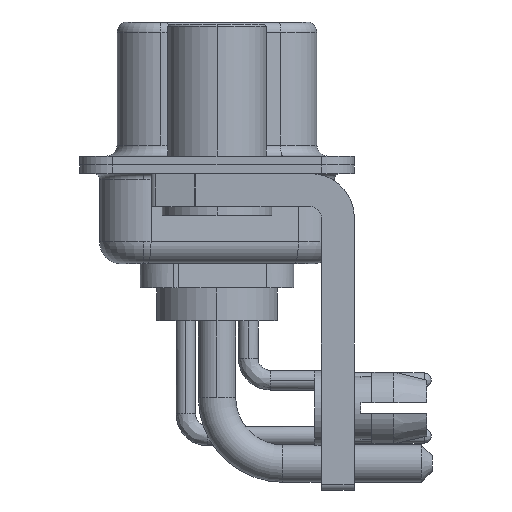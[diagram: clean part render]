
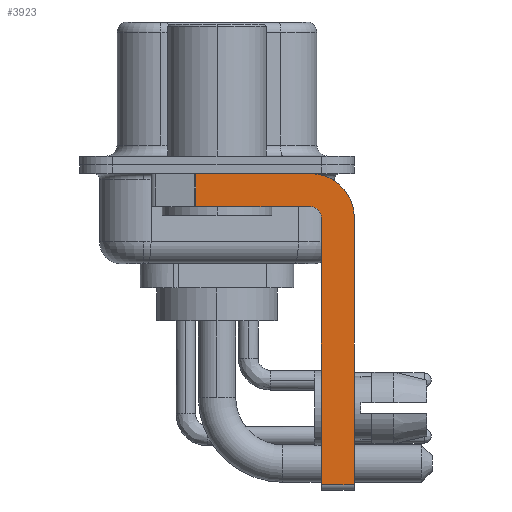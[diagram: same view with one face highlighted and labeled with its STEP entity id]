
A CAD part, left-side view. The second image highlights one B-rep face of the part: STEP entity #3923.
In plain terms, the highlighted planar face has unit normal (-1, 0, 0).
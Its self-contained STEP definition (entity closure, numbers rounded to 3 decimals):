
#31 = AXIS2_PLACEMENT_3D ( 'NONE', #22232, #9031, #4974 ) ;
#358 = VECTOR ( 'NONE', #23900, 1000. ) ;
#621 = EDGE_CURVE ( 'NONE', #6019, #10867, #24239, .T. ) ;
#1189 = LINE ( 'NONE', #20090, #23398 ) ;
#1366 = VERTEX_POINT ( 'NONE', #14848 ) ;
#1662 = DIRECTION ( 'NONE',  ( 0., 0., 1. ) ) ;
#2392 = AXIS2_PLACEMENT_3D ( 'NONE', #15628, #11678, #1662 ) ;
#2664 = LINE ( 'NONE', #11930, #7193 ) ;
#2903 = DIRECTION ( 'NONE',  ( 1., 0., 0. ) ) ;
#3574 = ORIENTED_EDGE ( 'NONE', *, *, #7593, .F. ) ;
#3923 = ADVANCED_FACE ( 'NONE', ( #22184 ), #6575, .F. ) ;
#4880 = CARTESIAN_POINT ( 'NONE',  ( -2.9, 3., -0.4 ) ) ;
#4974 = DIRECTION ( 'NONE',  ( 0., 0., -1. ) ) ;
#4986 = DIRECTION ( 'NONE',  ( 0., 1., 0. ) ) ;
#5110 = CARTESIAN_POINT ( 'NONE',  ( -2.9, -4.25, -1.9 ) ) ;
#5561 = DIRECTION ( 'NONE',  ( 0., 0., 1. ) ) ;
#6019 = VERTEX_POINT ( 'NONE', #6794 ) ;
#6575 = PLANE ( 'NONE',  #6641 ) ;
#6641 = AXIS2_PLACEMENT_3D ( 'NONE', #20277, #2903, #16482 ) ;
#6794 = CARTESIAN_POINT ( 'NONE',  ( -2.9, -4.75, -14.55 ) ) ;
#6993 = EDGE_CURVE ( 'NONE', #18891, #24413, #19817, .T. ) ;
#7193 = VECTOR ( 'NONE', #22077, 1000. ) ;
#7248 = EDGE_CURVE ( 'NONE', #1366, #14386, #2664, .T. ) ;
#7593 = EDGE_CURVE ( 'NONE', #6019, #18891, #18884, .T. ) ;
#8742 = ORIENTED_EDGE ( 'NONE', *, *, #6993, .F. ) ;
#9031 = DIRECTION ( 'NONE',  ( 1., 0., 0. ) ) ;
#9593 = CARTESIAN_POINT ( 'NONE',  ( -2.9, -4.75, -2.4 ) ) ;
#9919 = CARTESIAN_POINT ( 'NONE',  ( -2.9, -4.25, -0.4 ) ) ;
#10383 = ORIENTED_EDGE ( 'NONE', *, *, #7248, .T. ) ;
#10867 = VERTEX_POINT ( 'NONE', #16445 ) ;
#11344 = VECTOR ( 'NONE', #12627, 1000. ) ;
#11678 = DIRECTION ( 'NONE',  ( -1., 0., 0. ) ) ;
#11930 = CARTESIAN_POINT ( 'NONE',  ( -2.9, 0.978, -1.9 ) ) ;
#12595 = EDGE_CURVE ( 'NONE', #24413, #14386, #1189, .T. ) ;
#12627 = DIRECTION ( 'NONE',  ( 0., -1., 0. ) ) ;
#13892 = CARTESIAN_POINT ( 'NONE',  ( -2.9, -6.25, -2.4 ) ) ;
#13900 = ORIENTED_EDGE ( 'NONE', *, *, #19522, .F. ) ;
#14386 = VERTEX_POINT ( 'NONE', #22008 ) ;
#14742 = CARTESIAN_POINT ( 'NONE',  ( -2.9, -4.25, -14.55 ) ) ;
#14848 = CARTESIAN_POINT ( 'NONE',  ( -2.9, 0.978, -0.4 ) ) ;
#14945 = VERTEX_POINT ( 'NONE', #9919 ) ;
#15628 = CARTESIAN_POINT ( 'NONE',  ( -2.9, -4.25, -2.4 ) ) ;
#15629 = VERTEX_POINT ( 'NONE', #24347 ) ;
#16445 = CARTESIAN_POINT ( 'NONE',  ( -2.9, -6.25, -14.55 ) ) ;
#16455 = ORIENTED_EDGE ( 'NONE', *, *, #12595, .F. ) ;
#16482 = DIRECTION ( 'NONE',  ( 0., 0., -1. ) ) ;
#17550 = VECTOR ( 'NONE', #22091, 1000. ) ;
#17625 = ORIENTED_EDGE ( 'NONE', *, *, #17663, .F. ) ;
#17663 = EDGE_CURVE ( 'NONE', #15629, #10867, #21505, .T. ) ;
#18884 = LINE ( 'NONE', #23200, #22653 ) ;
#18891 = VERTEX_POINT ( 'NONE', #9593 ) ;
#19062 = ORIENTED_EDGE ( 'NONE', *, *, #621, .T. ) ;
#19522 = EDGE_CURVE ( 'NONE', #1366, #14945, #22260, .T. ) ;
#19817 = CIRCLE ( 'NONE', #2392, 0.5 ) ;
#19924 = EDGE_CURVE ( 'NONE', #14945, #15629, #22711, .T. ) ;
#20090 = CARTESIAN_POINT ( 'NONE',  ( -2.9, -4.25, -1.9 ) ) ;
#20277 = CARTESIAN_POINT ( 'NONE',  ( -2.9, -4.25, -2.4 ) ) ;
#20815 = ORIENTED_EDGE ( 'NONE', *, *, #19924, .F. ) ;
#21371 = EDGE_LOOP ( 'NONE', ( #13900, #10383, #16455, #8742, #3574, #19062, #17625, #20815 ) ) ;
#21505 = LINE ( 'NONE', #13892, #358 ) ;
#22008 = CARTESIAN_POINT ( 'NONE',  ( -2.9, 0.978, -1.9 ) ) ;
#22077 = DIRECTION ( 'NONE',  ( 0., 0., -1. ) ) ;
#22091 = DIRECTION ( 'NONE',  ( 0., -1., 0. ) ) ;
#22184 = FACE_OUTER_BOUND ( 'NONE', #21371, .T. ) ;
#22232 = CARTESIAN_POINT ( 'NONE',  ( -2.9, -4.25, -2.4 ) ) ;
#22260 = LINE ( 'NONE', #4880, #11344 ) ;
#22653 = VECTOR ( 'NONE', #5561, 1000. ) ;
#22711 = CIRCLE ( 'NONE', #31, 2. ) ;
#23200 = CARTESIAN_POINT ( 'NONE',  ( -2.9, -4.75, -14.8 ) ) ;
#23398 = VECTOR ( 'NONE', #4986, 1000. ) ;
#23900 = DIRECTION ( 'NONE',  ( 0., 0., -1. ) ) ;
#24239 = LINE ( 'NONE', #14742, #17550 ) ;
#24347 = CARTESIAN_POINT ( 'NONE',  ( -2.9, -6.25, -2.4 ) ) ;
#24413 = VERTEX_POINT ( 'NONE', #5110 ) ;
